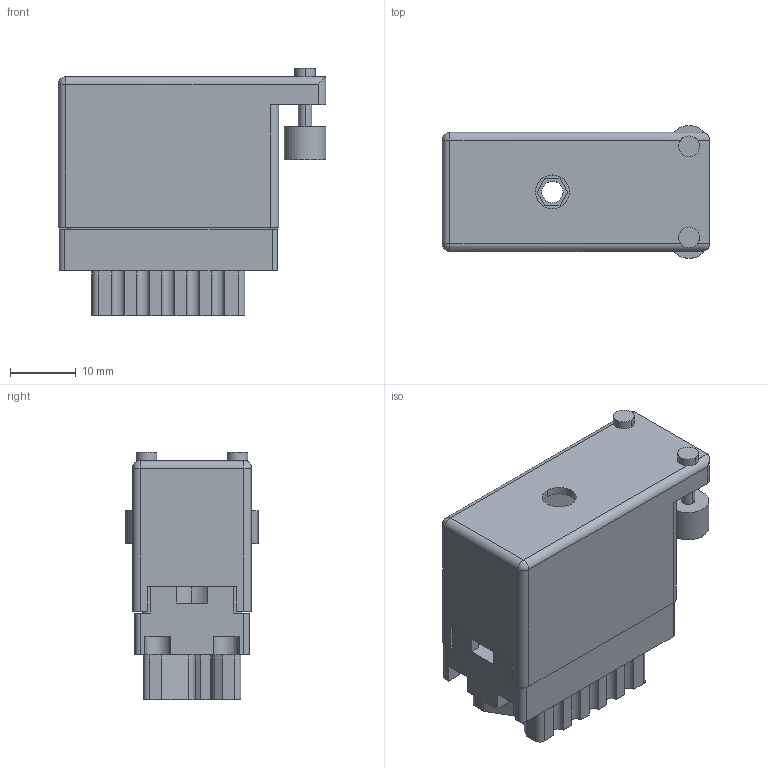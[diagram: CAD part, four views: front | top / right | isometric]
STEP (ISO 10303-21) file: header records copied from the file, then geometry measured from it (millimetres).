
FILE_DESCRIPTION (( 'STEP AP203' ), '1' );
FILE_NAME ('516-020-000-620.STEP', '2020-03-04T16:52:00', ( '' ), ( '' ), 'SwSTEP 2.0', 'SolidWorks 2016', '' );
FILE_SCHEMA (( 'CONFIG_CONTROL_DESIGN' ));
Length unit declared in the file: inch
Products named in the file (3): 516-020-000-620; 516 Part Receptacle_020; 516-230-001_Plastic - 020 Side Entry
Assembly tree (2 placements, depth 2):
  516-020-000-620
    516 Part Receptacle_020
    516-230-001_Plastic - 020 Side Entry
Bounding box: 40.87 x 20.24 x 37.77 mm (x, y, z)
Volume: 8901.9 mm3; surface area: 14417.4 mm2
Topology: 2 solids, 2 shells, 672 faces, 1964 edges, 1302 vertices
Faces by surface type: plane 446, cylinder 222, cone 2, sphere 2
Entity records: 22725 total; most frequent: CARTESIAN_POINT 3967, ORIENTED_EDGE 3924, DIRECTION 3842, EDGE_CURVE 1962, LINE 1424, VECTOR 1424, VERTEX_POINT 1302, AXIS2_PLACEMENT_3D 1209
